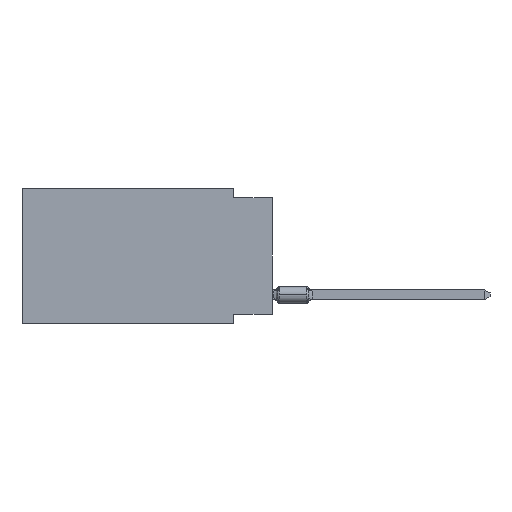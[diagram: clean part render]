
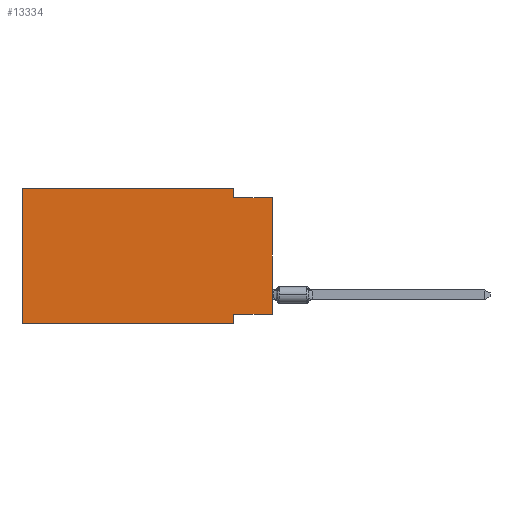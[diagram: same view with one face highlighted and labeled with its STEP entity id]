
A CAD part, left-side view. The second image highlights one B-rep face of the part: STEP entity #13334.
In plain terms, the highlighted planar face has unit normal (-1, 0, 0).
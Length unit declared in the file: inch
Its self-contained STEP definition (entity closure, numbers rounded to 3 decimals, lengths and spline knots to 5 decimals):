
#152 = ORIENTED_EDGE ( 'NONE', *, *, #16913, .F. ) ;
#160 = CARTESIAN_POINT ( 'NONE',  ( 0., 0.1, -0.35 ) ) ;
#608 = LINE ( 'NONE', #18569, #17661 ) ;
#725 = CARTESIAN_POINT ( 'NONE',  ( 0., 0., -0.025 ) ) ;
#2629 = CARTESIAN_POINT ( 'NONE',  ( 0., 0.1, -0.325 ) ) ;
#2680 = CARTESIAN_POINT ( 'NONE',  ( 0., 0.645, -0.35 ) ) ;
#3799 = EDGE_CURVE ( 'NONE', #17815, #12491, #36668, .T. ) ;
#4972 = CARTESIAN_POINT ( 'NONE',  ( 0., 0.645, 0. ) ) ;
#5552 = DIRECTION ( 'NONE',  ( 1., 0., 0. ) ) ;
#5598 = ORIENTED_EDGE ( 'NONE', *, *, #26754, .T. ) ;
#6601 = DIRECTION ( 'NONE',  ( 0., 0., 1. ) ) ;
#6645 = VERTEX_POINT ( 'NONE', #31623 ) ;
#7909 = CARTESIAN_POINT ( 'NONE',  ( 0., 0.1, 0. ) ) ;
#8360 = DIRECTION ( 'NONE',  ( 0., -1., 0. ) ) ;
#8400 = EDGE_CURVE ( 'NONE', #6645, #19242, #30509, .T. ) ;
#9330 = DIRECTION ( 'NONE',  ( 0., 0., -1. ) ) ;
#10055 = EDGE_LOOP ( 'NONE', ( #5598, #32026, #27373, #34361, #20219, #34426, #31025, #152 ) ) ;
#12238 = EDGE_CURVE ( 'NONE', #35886, #17815, #608, .T. ) ;
#12491 = VERTEX_POINT ( 'NONE', #34610 ) ;
#12604 = VECTOR ( 'NONE', #28321, 39.37008 ) ;
#12918 = CARTESIAN_POINT ( 'NONE',  ( 0., 0., -0.325 ) ) ;
#13251 = VERTEX_POINT ( 'NONE', #12918 ) ;
#13334 = ADVANCED_FACE ( 'NONE', ( #20072 ), #37655, .F. ) ;
#13785 = CARTESIAN_POINT ( 'NONE',  ( 0., 0.645, -0.35 ) ) ;
#15084 = AXIS2_PLACEMENT_3D ( 'NONE', #4972, #5552, #28756 ) ;
#15192 = VECTOR ( 'NONE', #19317, 39.37008 ) ;
#15197 = LINE ( 'NONE', #31874, #35869 ) ;
#16913 = EDGE_CURVE ( 'NONE', #13251, #21046, #15197, .T. ) ;
#17644 = VECTOR ( 'NONE', #8360, 39.37008 ) ;
#17661 = VECTOR ( 'NONE', #6601, 39.37008 ) ;
#17815 = VERTEX_POINT ( 'NONE', #19134 ) ;
#18569 = CARTESIAN_POINT ( 'NONE',  ( 0., 0.645, 0. ) ) ;
#18857 = EDGE_CURVE ( 'NONE', #21046, #19152, #28210, .T. ) ;
#18935 = CARTESIAN_POINT ( 'NONE',  ( 0., 0., -0.025 ) ) ;
#19002 = EDGE_CURVE ( 'NONE', #12491, #6645, #37868, .T. ) ;
#19134 = CARTESIAN_POINT ( 'NONE',  ( 0., 0.645, 0. ) ) ;
#19152 = VERTEX_POINT ( 'NONE', #160 ) ;
#19242 = VERTEX_POINT ( 'NONE', #725 ) ;
#19317 = DIRECTION ( 'NONE',  ( 0., -1., 0. ) ) ;
#20017 = LINE ( 'NONE', #28136, #12604 ) ;
#20072 = FACE_OUTER_BOUND ( 'NONE', #10055, .T. ) ;
#20219 = ORIENTED_EDGE ( 'NONE', *, *, #12238, .F. ) ;
#21046 = VERTEX_POINT ( 'NONE', #2629 ) ;
#21385 = DIRECTION ( 'NONE',  ( 0., 1., 0. ) ) ;
#22232 = CARTESIAN_POINT ( 'NONE',  ( 0., 0.1, -0.35 ) ) ;
#22327 = EDGE_CURVE ( 'NONE', #35886, #19152, #31176, .T. ) ;
#26754 = EDGE_CURVE ( 'NONE', #13251, #19242, #20017, .T. ) ;
#27373 = ORIENTED_EDGE ( 'NONE', *, *, #19002, .F. ) ;
#27395 = DIRECTION ( 'NONE',  ( 0., -1., 0. ) ) ;
#27594 = CARTESIAN_POINT ( 'NONE',  ( 0., 0.645, 0. ) ) ;
#28136 = CARTESIAN_POINT ( 'NONE',  ( 0., 0., 0. ) ) ;
#28210 = LINE ( 'NONE', #22232, #33525 ) ;
#28321 = DIRECTION ( 'NONE',  ( 0., 0., 1. ) ) ;
#28582 = DIRECTION ( 'NONE',  ( 0., 0., -1. ) ) ;
#28756 = DIRECTION ( 'NONE',  ( 0., 0., -1. ) ) ;
#30509 = LINE ( 'NONE', #18935, #15192 ) ;
#31025 = ORIENTED_EDGE ( 'NONE', *, *, #18857, .F. ) ;
#31176 = LINE ( 'NONE', #13785, #17644 ) ;
#31623 = CARTESIAN_POINT ( 'NONE',  ( 0., 0.1, -0.025 ) ) ;
#31676 = VECTOR ( 'NONE', #28582, 39.37008 ) ;
#31874 = CARTESIAN_POINT ( 'NONE',  ( 0., 0., -0.325 ) ) ;
#32026 = ORIENTED_EDGE ( 'NONE', *, *, #8400, .F. ) ;
#33525 = VECTOR ( 'NONE', #9330, 39.37008 ) ;
#34361 = ORIENTED_EDGE ( 'NONE', *, *, #3799, .F. ) ;
#34426 = ORIENTED_EDGE ( 'NONE', *, *, #22327, .T. ) ;
#34610 = CARTESIAN_POINT ( 'NONE',  ( 0., 0.1, 0. ) ) ;
#35869 = VECTOR ( 'NONE', #21385, 39.37008 ) ;
#35886 = VERTEX_POINT ( 'NONE', #2680 ) ;
#36668 = LINE ( 'NONE', #27594, #37102 ) ;
#37102 = VECTOR ( 'NONE', #27395, 39.37008 ) ;
#37655 = PLANE ( 'NONE',  #15084 ) ;
#37868 = LINE ( 'NONE', #7909, #31676 ) ;
